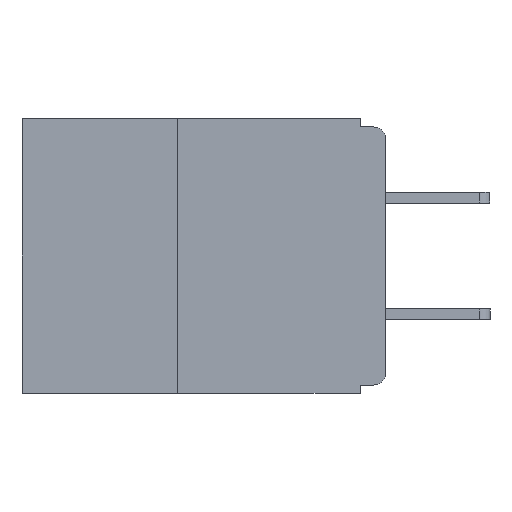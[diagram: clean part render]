
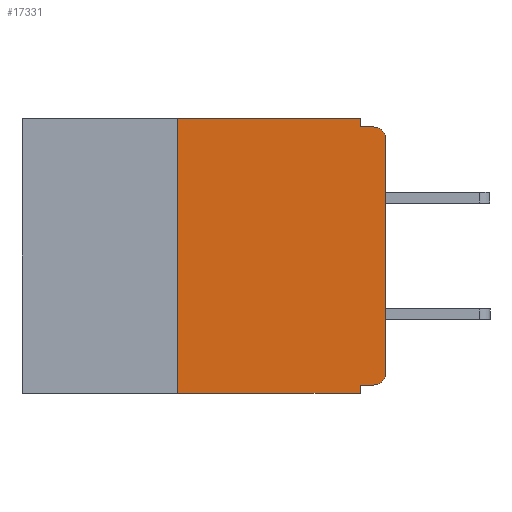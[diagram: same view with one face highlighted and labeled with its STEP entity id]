
A CAD part, left-side view. The second image highlights one B-rep face of the part: STEP entity #17331.
In plain terms, the highlighted planar face has unit normal (-1, 0, 0).
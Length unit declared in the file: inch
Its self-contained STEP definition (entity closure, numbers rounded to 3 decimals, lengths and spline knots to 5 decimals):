
#38 = VERTEX_POINT ( 'NONE', #26415 ) ;
#560 = CARTESIAN_POINT ( 'NONE',  ( 0., 0.015, -0.025 ) ) ;
#581 = CARTESIAN_POINT ( 'NONE',  ( 0., 0., -0.01 ) ) ;
#660 = ORIENTED_EDGE ( 'NONE', *, *, #12299, .T. ) ;
#737 = VERTEX_POINT ( 'NONE', #9274 ) ;
#998 = VECTOR ( 'NONE', #21552, 39.37008 ) ;
#1049 = CARTESIAN_POINT ( 'NONE',  ( 0., 0.031, -0.33 ) ) ;
#1236 = EDGE_CURVE ( 'NONE', #4534, #38, #1286, .T. ) ;
#1286 = CIRCLE ( 'NONE', #7518, 0.015 ) ;
#1312 = VECTOR ( 'NONE', #27801, 39.37008 ) ;
#1573 = DIRECTION ( 'NONE',  ( 0., 1., 0. ) ) ;
#1634 = VERTEX_POINT ( 'NONE', #26075 ) ;
#1945 = ORIENTED_EDGE ( 'NONE', *, *, #13804, .T. ) ;
#1966 = EDGE_CURVE ( 'NONE', #4757, #21837, #5568, .T. ) ;
#2346 = CIRCLE ( 'NONE', #27015, 0.015 ) ;
#2619 = DIRECTION ( 'NONE',  ( 0., -1., 0. ) ) ;
#2913 = DIRECTION ( 'NONE',  ( 0., 0., -1. ) ) ;
#3312 = VECTOR ( 'NONE', #15135, 39.37008 ) ;
#4534 = VERTEX_POINT ( 'NONE', #19791 ) ;
#4613 = ORIENTED_EDGE ( 'NONE', *, *, #20598, .F. ) ;
#4757 = VERTEX_POINT ( 'NONE', #29381 ) ;
#5359 = CARTESIAN_POINT ( 'NONE',  ( 0., 0.031, 0. ) ) ;
#5404 = PLANE ( 'NONE',  #15831 ) ;
#5568 = LINE ( 'NONE', #5848, #16993 ) ;
#5643 = DIRECTION ( 'NONE',  ( 0., -1., 0. ) ) ;
#5848 = CARTESIAN_POINT ( 'NONE',  ( 0., 0.437, 0. ) ) ;
#6070 = EDGE_CURVE ( 'NONE', #15309, #737, #13515, .T. ) ;
#6346 = EDGE_CURVE ( 'NONE', #11609, #6561, #17806, .T. ) ;
#6416 = FACE_OUTER_BOUND ( 'NONE', #11019, .T. ) ;
#6561 = VERTEX_POINT ( 'NONE', #12437 ) ;
#6664 = EDGE_CURVE ( 'NONE', #21837, #15309, #26538, .T. ) ;
#7150 = ORIENTED_EDGE ( 'NONE', *, *, #6070, .F. ) ;
#7518 = AXIS2_PLACEMENT_3D ( 'NONE', #14180, #14129, #14026 ) ;
#7732 = DIRECTION ( 'NONE',  ( 0., 0., -1. ) ) ;
#8736 = LINE ( 'NONE', #12854, #3312 ) ;
#9274 = CARTESIAN_POINT ( 'NONE',  ( 0., 0.015, -0.01 ) ) ;
#9477 = CARTESIAN_POINT ( 'NONE',  ( 0., 0.437, -0.33 ) ) ;
#10412 = ORIENTED_EDGE ( 'NONE', *, *, #1236, .T. ) ;
#10541 = DIRECTION ( 'NONE',  ( 0., 0., -1. ) ) ;
#10659 = LINE ( 'NONE', #26326, #15980 ) ;
#10835 = CARTESIAN_POINT ( 'NONE',  ( 0., 0., -0.32 ) ) ;
#10925 = ORIENTED_EDGE ( 'NONE', *, *, #6346, .T. ) ;
#11019 = EDGE_LOOP ( 'NONE', ( #1945, #660, #7150, #27998, #16616, #4613, #10925, #28172, #11715, #10412 ) ) ;
#11609 = VERTEX_POINT ( 'NONE', #28709 ) ;
#11715 = ORIENTED_EDGE ( 'NONE', *, *, #23235, .F. ) ;
#12080 = CARTESIAN_POINT ( 'NONE',  ( 0., 0.031, -0.32 ) ) ;
#12299 = EDGE_CURVE ( 'NONE', #1634, #737, #2346, .T. ) ;
#12437 = CARTESIAN_POINT ( 'NONE',  ( 0., 0.031, -0.33 ) ) ;
#12854 = CARTESIAN_POINT ( 'NONE',  ( 0., 0., 0. ) ) ;
#13515 = LINE ( 'NONE', #581, #1312 ) ;
#13804 = EDGE_CURVE ( 'NONE', #38, #1634, #8736, .T. ) ;
#14026 = DIRECTION ( 'NONE',  ( 0., 0., -1. ) ) ;
#14129 = DIRECTION ( 'NONE',  ( -1., 0., 0. ) ) ;
#14180 = CARTESIAN_POINT ( 'NONE',  ( 0., 0.015, -0.305 ) ) ;
#14339 = CARTESIAN_POINT ( 'NONE',  ( 0., 0.031, -0.01 ) ) ;
#14524 = CARTESIAN_POINT ( 'NONE',  ( 0., 0.437, 0. ) ) ;
#15135 = DIRECTION ( 'NONE',  ( 0., 0., 1. ) ) ;
#15309 = VERTEX_POINT ( 'NONE', #14339 ) ;
#15455 = LINE ( 'NONE', #10835, #20784 ) ;
#15831 = AXIS2_PLACEMENT_3D ( 'NONE', #14524, #21378, #7732 ) ;
#15980 = VECTOR ( 'NONE', #28614, 39.37008 ) ;
#16114 = EDGE_CURVE ( 'NONE', #28289, #6561, #25225, .T. ) ;
#16601 = DIRECTION ( 'NONE',  ( -1., 0., 0. ) ) ;
#16616 = ORIENTED_EDGE ( 'NONE', *, *, #1966, .F. ) ;
#16993 = VECTOR ( 'NONE', #5643, 39.37008 ) ;
#17331 = ADVANCED_FACE ( 'NONE', ( #6416 ), #5404, .F. ) ;
#17806 = LINE ( 'NONE', #9477, #28947 ) ;
#19791 = CARTESIAN_POINT ( 'NONE',  ( 0., 0.015, -0.32 ) ) ;
#20591 = VECTOR ( 'NONE', #10541, 39.37008 ) ;
#20598 = EDGE_CURVE ( 'NONE', #11609, #4757, #10659, .T. ) ;
#20784 = VECTOR ( 'NONE', #1573, 39.37008 ) ;
#21378 = DIRECTION ( 'NONE',  ( 1., 0., 0. ) ) ;
#21552 = DIRECTION ( 'NONE',  ( 0., 0., -1. ) ) ;
#21837 = VERTEX_POINT ( 'NONE', #5359 ) ;
#21893 = CARTESIAN_POINT ( 'NONE',  ( 0., 0.031, 0. ) ) ;
#23235 = EDGE_CURVE ( 'NONE', #4534, #28289, #15455, .T. ) ;
#25225 = LINE ( 'NONE', #1049, #998 ) ;
#26075 = CARTESIAN_POINT ( 'NONE',  ( 0., 0., -0.025 ) ) ;
#26326 = CARTESIAN_POINT ( 'NONE',  ( 0., 0.25, -0.33 ) ) ;
#26415 = CARTESIAN_POINT ( 'NONE',  ( 0., 0., -0.305 ) ) ;
#26538 = LINE ( 'NONE', #21893, #20591 ) ;
#27015 = AXIS2_PLACEMENT_3D ( 'NONE', #560, #16601, #2913 ) ;
#27801 = DIRECTION ( 'NONE',  ( 0., -1., 0. ) ) ;
#27998 = ORIENTED_EDGE ( 'NONE', *, *, #6664, .F. ) ;
#28172 = ORIENTED_EDGE ( 'NONE', *, *, #16114, .F. ) ;
#28289 = VERTEX_POINT ( 'NONE', #12080 ) ;
#28614 = DIRECTION ( 'NONE',  ( 0., 0., 1. ) ) ;
#28709 = CARTESIAN_POINT ( 'NONE',  ( 0., 0.25, -0.33 ) ) ;
#28947 = VECTOR ( 'NONE', #2619, 39.37008 ) ;
#29381 = CARTESIAN_POINT ( 'NONE',  ( 0., 0.25, 0. ) ) ;
